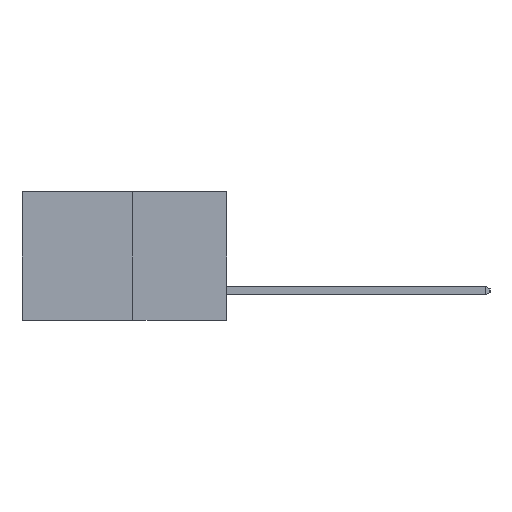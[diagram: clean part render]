
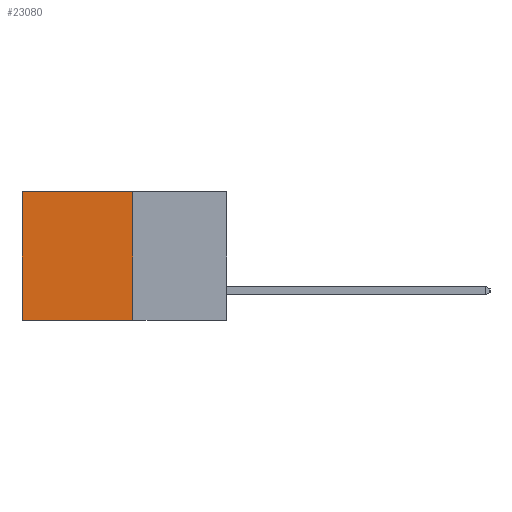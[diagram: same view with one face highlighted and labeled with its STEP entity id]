
A CAD part, left-side view. The second image highlights one B-rep face of the part: STEP entity #23080.
In plain terms, the highlighted planar face has unit normal (-1, 0, 0).
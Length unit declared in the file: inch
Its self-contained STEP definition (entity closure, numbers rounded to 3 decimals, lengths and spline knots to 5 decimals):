
#364 = LINE ( 'NONE', #24277, #11481 ) ;
#929 = EDGE_CURVE ( 'NONE', #12110, #18742, #11093, .T. ) ;
#1937 = DIRECTION ( 'NONE',  ( 0., 1., 0. ) ) ;
#3714 = EDGE_LOOP ( 'NONE', ( #10483, #13661, #11274, #25541 ) ) ;
#3767 = DIRECTION ( 'NONE',  ( 0., 0., -1. ) ) ;
#4163 = DIRECTION ( 'NONE',  ( 0., 1., 0. ) ) ;
#5214 = VECTOR ( 'NONE', #3767, 39.37008 ) ;
#6394 = AXIS2_PLACEMENT_3D ( 'NONE', #8913, #11136, #26135 ) ;
#6439 = LINE ( 'NONE', #19581, #23161 ) ;
#8625 = CARTESIAN_POINT ( 'NONE',  ( 0.277, 0.59, -0.37 ) ) ;
#8913 = CARTESIAN_POINT ( 'NONE',  ( 0.277, 0.27, -0.37 ) ) ;
#9916 = LINE ( 'NONE', #12983, #26360 ) ;
#10483 = ORIENTED_EDGE ( 'NONE', *, *, #929, .T. ) ;
#10608 = EDGE_CURVE ( 'NONE', #20792, #12110, #6439, .T. ) ;
#11093 = LINE ( 'NONE', #8625, #5214 ) ;
#11136 = DIRECTION ( 'NONE',  ( 1., 0., 0. ) ) ;
#11274 = ORIENTED_EDGE ( 'NONE', *, *, #22792, .F. ) ;
#11481 = VECTOR ( 'NONE', #26342, 39.37008 ) ;
#11689 = CARTESIAN_POINT ( 'NONE',  ( 0.277, 0.27, -0.37 ) ) ;
#12110 = VERTEX_POINT ( 'NONE', #13131 ) ;
#12983 = CARTESIAN_POINT ( 'NONE',  ( 0.277, 0.27, -0.37 ) ) ;
#12997 = CARTESIAN_POINT ( 'NONE',  ( 0.277, 0.27, 0. ) ) ;
#13131 = CARTESIAN_POINT ( 'NONE',  ( 0.277, 0.59, 0. ) ) ;
#13661 = ORIENTED_EDGE ( 'NONE', *, *, #17205, .F. ) ;
#14221 = FACE_OUTER_BOUND ( 'NONE', #3714, .T. ) ;
#17205 = EDGE_CURVE ( 'NONE', #21683, #18742, #9916, .T. ) ;
#18742 = VERTEX_POINT ( 'NONE', #20092 ) ;
#19581 = CARTESIAN_POINT ( 'NONE',  ( 0.277, 0.27, 0. ) ) ;
#20092 = CARTESIAN_POINT ( 'NONE',  ( 0.277, 0.59, -0.37 ) ) ;
#20792 = VERTEX_POINT ( 'NONE', #12997 ) ;
#21683 = VERTEX_POINT ( 'NONE', #11689 ) ;
#21987 = PLANE ( 'NONE',  #6394 ) ;
#22792 = EDGE_CURVE ( 'NONE', #20792, #21683, #364, .T. ) ;
#23080 = ADVANCED_FACE ( 'NONE', ( #14221 ), #21987, .F. ) ;
#23161 = VECTOR ( 'NONE', #4163, 39.37008 ) ;
#24277 = CARTESIAN_POINT ( 'NONE',  ( 0.277, 0.27, -0.37 ) ) ;
#25541 = ORIENTED_EDGE ( 'NONE', *, *, #10608, .T. ) ;
#26135 = DIRECTION ( 'NONE',  ( 0., 0., -1. ) ) ;
#26342 = DIRECTION ( 'NONE',  ( 0., 0., -1. ) ) ;
#26360 = VECTOR ( 'NONE', #1937, 39.37008 ) ;
